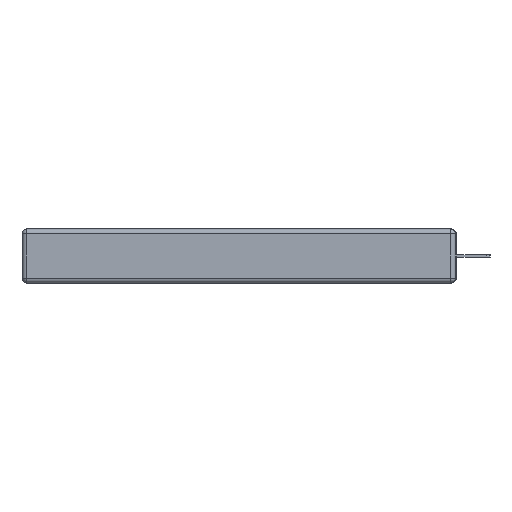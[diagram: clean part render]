
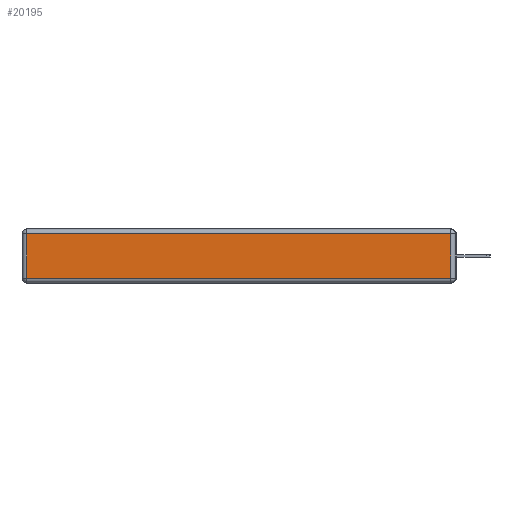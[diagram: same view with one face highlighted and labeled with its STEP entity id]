
A CAD part, left-side view. The second image highlights one B-rep face of the part: STEP entity #20195.
In plain terms, the highlighted planar face has unit normal (-1, 0, 0).
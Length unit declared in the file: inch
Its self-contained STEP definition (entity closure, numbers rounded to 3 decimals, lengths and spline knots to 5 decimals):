
#298 = DIRECTION ( 'NONE',  ( 0., 0., 1. ) ) ;
#1097 = VERTEX_POINT ( 'NONE', #17646 ) ;
#1857 = CARTESIAN_POINT ( 'NONE',  ( 0., 2.72, -0.03 ) ) ;
#3256 = VERTEX_POINT ( 'NONE', #1857 ) ;
#3361 = LINE ( 'NONE', #17216, #5999 ) ;
#3419 = DIRECTION ( 'NONE',  ( -1., 0., 0. ) ) ;
#4072 = CARTESIAN_POINT ( 'NONE',  ( 0., 0.03, -0.343 ) ) ;
#4527 = EDGE_CURVE ( 'NONE', #16886, #1097, #19383, .T. ) ;
#5519 = CARTESIAN_POINT ( 'NONE',  ( 0., 0., -0.313 ) ) ;
#5999 = VECTOR ( 'NONE', #24821, 39.37008 ) ;
#6093 = VECTOR ( 'NONE', #9458, 39.37008 ) ;
#6587 = ORIENTED_EDGE ( 'NONE', *, *, #15339, .T. ) ;
#7415 = CARTESIAN_POINT ( 'NONE',  ( 0., 2.75, -0.03 ) ) ;
#7555 = VECTOR ( 'NONE', #298, 39.37008 ) ;
#8103 = AXIS2_PLACEMENT_3D ( 'NONE', #23556, #3419, #9569 ) ;
#9458 = DIRECTION ( 'NONE',  ( 0., -1., 0. ) ) ;
#9569 = DIRECTION ( 'NONE',  ( 0., 0., 1. ) ) ;
#9947 = EDGE_LOOP ( 'NONE', ( #13926, #6587, #25582, #23500 ) ) ;
#13926 = ORIENTED_EDGE ( 'NONE', *, *, #4527, .T. ) ;
#14397 = LINE ( 'NONE', #4072, #7555 ) ;
#14536 = VERTEX_POINT ( 'NONE', #14856 ) ;
#14856 = CARTESIAN_POINT ( 'NONE',  ( 0., 0.03, -0.03 ) ) ;
#15339 = EDGE_CURVE ( 'NONE', #1097, #14536, #14397, .T. ) ;
#15389 = DIRECTION ( 'NONE',  ( 0., 1., 0. ) ) ;
#16440 = VECTOR ( 'NONE', #15389, 39.37008 ) ;
#16886 = VERTEX_POINT ( 'NONE', #25638 ) ;
#17216 = CARTESIAN_POINT ( 'NONE',  ( 0., 2.72, -0.343 ) ) ;
#17646 = CARTESIAN_POINT ( 'NONE',  ( 0., 0.03, -0.313 ) ) ;
#19115 = FACE_OUTER_BOUND ( 'NONE', #9947, .T. ) ;
#19378 = EDGE_CURVE ( 'NONE', #14536, #3256, #21261, .T. ) ;
#19383 = LINE ( 'NONE', #5519, #6093 ) ;
#20195 = ADVANCED_FACE ( 'NONE', ( #19115 ), #25645, .T. ) ;
#20473 = EDGE_CURVE ( 'NONE', #3256, #16886, #3361, .T. ) ;
#21261 = LINE ( 'NONE', #7415, #16440 ) ;
#23500 = ORIENTED_EDGE ( 'NONE', *, *, #20473, .T. ) ;
#23556 = CARTESIAN_POINT ( 'NONE',  ( 0., 0., -0.343 ) ) ;
#24821 = DIRECTION ( 'NONE',  ( 0., 0., -1. ) ) ;
#25582 = ORIENTED_EDGE ( 'NONE', *, *, #19378, .T. ) ;
#25638 = CARTESIAN_POINT ( 'NONE',  ( 0., 2.72, -0.313 ) ) ;
#25645 = PLANE ( 'NONE',  #8103 ) ;
